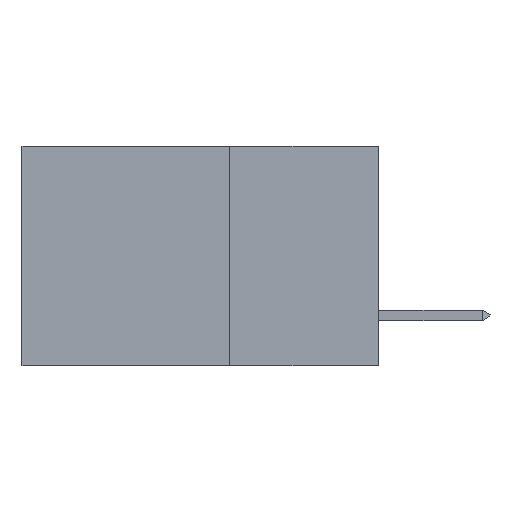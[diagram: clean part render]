
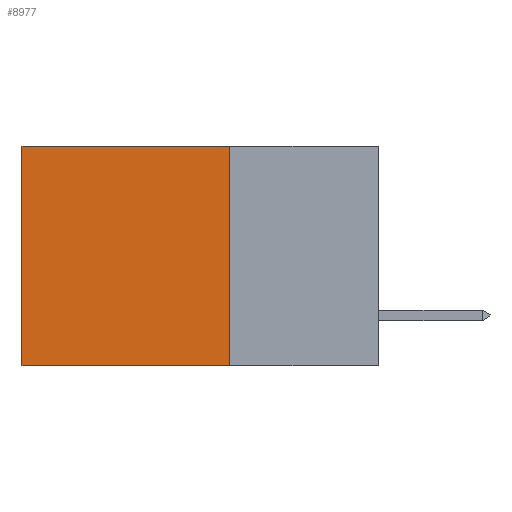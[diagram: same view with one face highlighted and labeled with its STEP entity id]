
A CAD part, left-side view. The second image highlights one B-rep face of the part: STEP entity #8977.
In plain terms, the highlighted planar face has unit normal (-1, 0, 0).
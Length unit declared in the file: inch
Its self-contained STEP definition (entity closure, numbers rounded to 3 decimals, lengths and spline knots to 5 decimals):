
#497 = EDGE_CURVE ( 'NONE', #2212, #17132, #5716, .T. ) ;
#512 = CARTESIAN_POINT ( 'NONE',  ( 0.298, 0.25, 0. ) ) ;
#747 = LINE ( 'NONE', #15083, #13887 ) ;
#898 = LINE ( 'NONE', #16764, #9060 ) ;
#1752 = CARTESIAN_POINT ( 'NONE',  ( 0.298, 0.25, 0. ) ) ;
#1890 = DIRECTION ( 'NONE',  ( 1., 0., 0. ) ) ;
#2053 = VECTOR ( 'NONE', #7958, 39.37008 ) ;
#2212 = VERTEX_POINT ( 'NONE', #16417 ) ;
#2316 = EDGE_LOOP ( 'NONE', ( #4329, #6020, #2364, #16423 ) ) ;
#2364 = ORIENTED_EDGE ( 'NONE', *, *, #497, .F. ) ;
#2665 = DIRECTION ( 'NONE',  ( 0., 1., 0. ) ) ;
#3135 = EDGE_CURVE ( 'NONE', #2212, #11584, #898, .T. ) ;
#3188 = PLANE ( 'NONE',  #5886 ) ;
#3249 = DIRECTION ( 'NONE',  ( 0., 0., -1. ) ) ;
#4280 = DIRECTION ( 'NONE',  ( 0., 1., 0. ) ) ;
#4329 = ORIENTED_EDGE ( 'NONE', *, *, #15913, .T. ) ;
#5270 = CARTESIAN_POINT ( 'NONE',  ( 0.298, 0.6, -0.37 ) ) ;
#5716 = LINE ( 'NONE', #1752, #17774 ) ;
#5886 = AXIS2_PLACEMENT_3D ( 'NONE', #512, #1890, #3249 ) ;
#6020 = ORIENTED_EDGE ( 'NONE', *, *, #16538, .F. ) ;
#7958 = DIRECTION ( 'NONE',  ( 0., 0., -1. ) ) ;
#8977 = ADVANCED_FACE ( 'NONE', ( #9358 ), #3188, .F. ) ;
#9060 = VECTOR ( 'NONE', #4280, 39.37008 ) ;
#9358 = FACE_OUTER_BOUND ( 'NONE', #2316, .T. ) ;
#9928 = DIRECTION ( 'NONE',  ( 0., 0., -1. ) ) ;
#10731 = CARTESIAN_POINT ( 'NONE',  ( 0.298, 0.6, 0. ) ) ;
#11039 = VERTEX_POINT ( 'NONE', #5270 ) ;
#11584 = VERTEX_POINT ( 'NONE', #14795 ) ;
#13047 = CARTESIAN_POINT ( 'NONE',  ( 0.298, 0.25, -0.37 ) ) ;
#13887 = VECTOR ( 'NONE', #2665, 39.37008 ) ;
#14754 = LINE ( 'NONE', #10731, #2053 ) ;
#14795 = CARTESIAN_POINT ( 'NONE',  ( 0.298, 0.6, 0. ) ) ;
#15083 = CARTESIAN_POINT ( 'NONE',  ( 0.298, 0.25, -0.37 ) ) ;
#15913 = EDGE_CURVE ( 'NONE', #11584, #11039, #14754, .T. ) ;
#16417 = CARTESIAN_POINT ( 'NONE',  ( 0.298, 0.25, 0. ) ) ;
#16423 = ORIENTED_EDGE ( 'NONE', *, *, #3135, .T. ) ;
#16538 = EDGE_CURVE ( 'NONE', #17132, #11039, #747, .T. ) ;
#16764 = CARTESIAN_POINT ( 'NONE',  ( 0.298, 0.25, 0. ) ) ;
#17132 = VERTEX_POINT ( 'NONE', #13047 ) ;
#17774 = VECTOR ( 'NONE', #9928, 39.37008 ) ;
